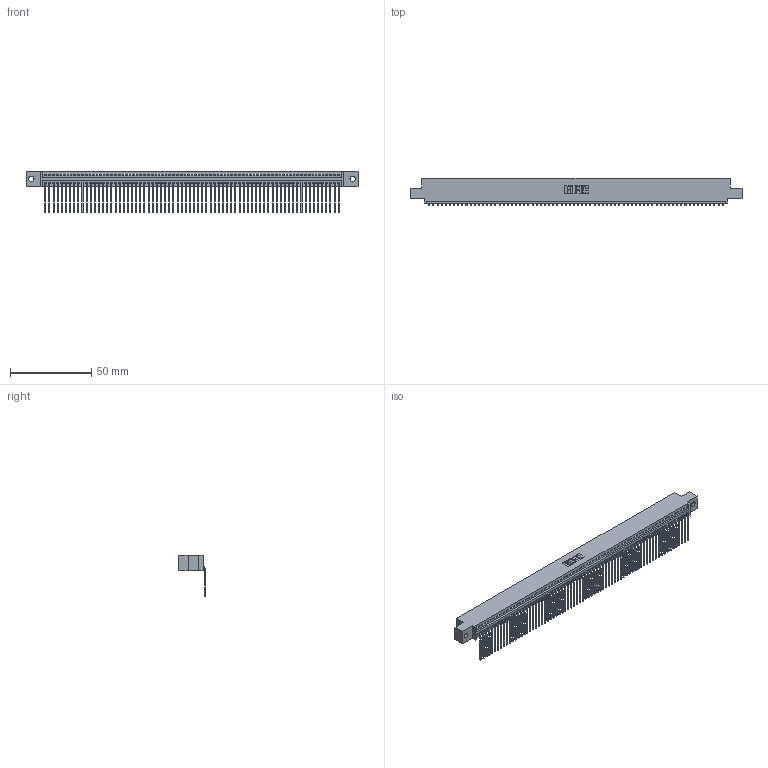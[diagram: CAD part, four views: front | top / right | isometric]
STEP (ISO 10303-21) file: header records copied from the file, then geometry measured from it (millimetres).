
FILE_DESCRIPTION (( 'STEP AP203' ), '1' );
FILE_NAME ('395-072-559-402.STEP', '2019-10-26T11:54:02', ( '' ), ( '' ), 'SwSTEP 2.0', 'SolidWorks 2016', '' );
FILE_SCHEMA (( 'CONFIG_CONTROL_DESIGN' ));
Length unit declared in the file: inch
Products named in the file (3): 395-072-559-402; 345-292-001_558 559 Tail - 1; 345 Part_0.110 Offset - 0.128 Dia
Assembly tree (73 placements, depth 2):
  395-072-559-402
    345 Part_0.110 Offset - 0.128 Dia
    345-292-001_558 559 Tail - 1  x72
Bounding box: 204.09 x 16.75 x 25.53 mm (x, y, z)
Volume: 19760.2 mm3; surface area: 27887.2 mm2
Topology: 73 solids, 73 shells, 4450 faces, 13457 edges, 8874 vertices
Faces by surface type: plane 3108, cylinder 1342
Entity records: 50369 total; most frequent: ORIENTED_EDGE 8738, CARTESIAN_POINT 8732, DIRECTION 7581, EDGE_CURVE 4369, LINE 3949, VECTOR 3949, VERTEX_POINT 2910, AXIS2_PLACEMENT_3D 1816
